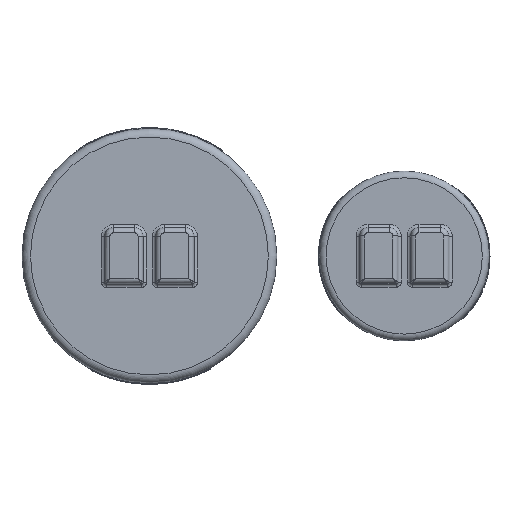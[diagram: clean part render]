
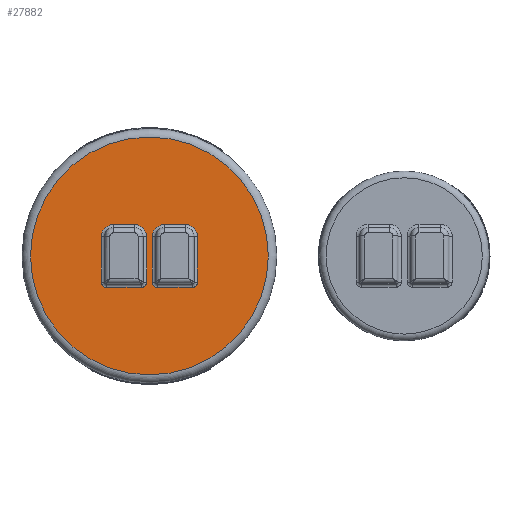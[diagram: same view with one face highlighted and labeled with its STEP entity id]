
A CAD part, top view. The second image highlights one B-rep face of the part: STEP entity #27882.
In plain terms, the highlighted planar face has unit normal (0, 0, 1).
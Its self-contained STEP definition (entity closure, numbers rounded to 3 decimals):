
#3316=FACE_BOUND('',#9538,.T.);
#3317=FACE_BOUND('',#9539,.T.);
#3658=PLANE('',#29710);
#4695=LINE('',#64399,#6189);
#4697=LINE('',#64411,#6191);
#4699=LINE('',#64423,#6193);
#4700=LINE('',#64431,#6194);
#4709=LINE('',#64458,#6203);
#4710=LINE('',#64462,#6204);
#4711=LINE('',#64466,#6205);
#4712=LINE('',#64469,#6206);
#6189=VECTOR('',#33431,10.);
#6191=VECTOR('',#33445,10.);
#6193=VECTOR('',#33459,10.);
#6194=VECTOR('',#33470,10.);
#6203=VECTOR('',#33497,10.);
#6204=VECTOR('',#33500,10.);
#6205=VECTOR('',#33503,10.);
#6206=VECTOR('',#33506,10.);
#7891=FACE_OUTER_BOUND('',#9537,.T.);
#9537=EDGE_LOOP('',(#22693));
#9538=EDGE_LOOP('',(#22694,#22695,#22696,#22697,#22698,#22699,#22700,#22701));
#9539=EDGE_LOOP('',(#22702,#22703,#22704,#22705,#22706,#22707,#22708,#22709));
#10638=CIRCLE('',#29682,7.);
#10644=CIRCLE('',#29690,7.);
#10648=CIRCLE('',#29696,3.);
#10652=CIRCLE('',#29702,3.);
#10655=CIRCLE('',#29711,70.);
#10656=CIRCLE('',#29712,7.);
#10657=CIRCLE('',#29713,3.);
#10658=CIRCLE('',#29714,3.);
#10659=CIRCLE('',#29715,7.);
#12360=VERTEX_POINT('',#64387);
#12361=VERTEX_POINT('',#64389);
#12363=VERTEX_POINT('',#64395);
#12365=VERTEX_POINT('',#64401);
#12367=VERTEX_POINT('',#64407);
#12369=VERTEX_POINT('',#64413);
#12371=VERTEX_POINT('',#64419);
#12373=VERTEX_POINT('',#64425);
#12380=VERTEX_POINT('',#64452);
#12381=VERTEX_POINT('',#64454);
#12382=VERTEX_POINT('',#64455);
#12383=VERTEX_POINT('',#64457);
#12384=VERTEX_POINT('',#64459);
#12385=VERTEX_POINT('',#64461);
#12386=VERTEX_POINT('',#64463);
#12387=VERTEX_POINT('',#64465);
#12388=VERTEX_POINT('',#64467);
#16025=EDGE_CURVE('',#12360,#12361,#10638,.T.);
#16030=EDGE_CURVE('',#12361,#12363,#4695,.T.);
#16033=EDGE_CURVE('',#12363,#12365,#10644,.T.);
#16036=EDGE_CURVE('',#12365,#12367,#4697,.T.);
#16039=EDGE_CURVE('',#12367,#12369,#10648,.T.);
#16042=EDGE_CURVE('',#12369,#12371,#4699,.T.);
#16045=EDGE_CURVE('',#12371,#12373,#10652,.T.);
#16046=EDGE_CURVE('',#12373,#12360,#4700,.T.);
#16057=EDGE_CURVE('',#12380,#12380,#10655,.T.);
#16058=EDGE_CURVE('',#12381,#12382,#10656,.T.);
#16059=EDGE_CURVE('',#12383,#12381,#4709,.T.);
#16060=EDGE_CURVE('',#12384,#12383,#10657,.T.);
#16061=EDGE_CURVE('',#12385,#12384,#4710,.T.);
#16062=EDGE_CURVE('',#12386,#12385,#10658,.T.);
#16063=EDGE_CURVE('',#12387,#12386,#4711,.T.);
#16064=EDGE_CURVE('',#12388,#12387,#10659,.T.);
#16065=EDGE_CURVE('',#12382,#12388,#4712,.T.);
#22693=ORIENTED_EDGE('',*,*,#16057,.F.);
#22694=ORIENTED_EDGE('',*,*,#16058,.F.);
#22695=ORIENTED_EDGE('',*,*,#16059,.F.);
#22696=ORIENTED_EDGE('',*,*,#16060,.F.);
#22697=ORIENTED_EDGE('',*,*,#16061,.F.);
#22698=ORIENTED_EDGE('',*,*,#16062,.F.);
#22699=ORIENTED_EDGE('',*,*,#16063,.F.);
#22700=ORIENTED_EDGE('',*,*,#16064,.F.);
#22701=ORIENTED_EDGE('',*,*,#16065,.F.);
#22702=ORIENTED_EDGE('',*,*,#16025,.F.);
#22703=ORIENTED_EDGE('',*,*,#16046,.F.);
#22704=ORIENTED_EDGE('',*,*,#16045,.F.);
#22705=ORIENTED_EDGE('',*,*,#16042,.F.);
#22706=ORIENTED_EDGE('',*,*,#16039,.F.);
#22707=ORIENTED_EDGE('',*,*,#16036,.F.);
#22708=ORIENTED_EDGE('',*,*,#16033,.F.);
#22709=ORIENTED_EDGE('',*,*,#16030,.F.);
#27882=ADVANCED_FACE('',(#7891,#3316,#3317),#3658,.T.);
#29682=AXIS2_PLACEMENT_3D('',#64390,#33420,#33421);
#29690=AXIS2_PLACEMENT_3D('',#64405,#33438,#33439);
#29696=AXIS2_PLACEMENT_3D('',#64417,#33452,#33453);
#29702=AXIS2_PLACEMENT_3D('',#64429,#33466,#33467);
#29710=AXIS2_PLACEMENT_3D('',#64451,#33491,#33492);
#29711=AXIS2_PLACEMENT_3D('',#64453,#33493,#33494);
#29712=AXIS2_PLACEMENT_3D('',#64456,#33495,#33496);
#29713=AXIS2_PLACEMENT_3D('',#64460,#33498,#33499);
#29714=AXIS2_PLACEMENT_3D('',#64464,#33501,#33502);
#29715=AXIS2_PLACEMENT_3D('',#64468,#33504,#33505);
#33420=DIRECTION('center_axis',(0.,0.,1.));
#33421=DIRECTION('ref_axis',(0.707,0.707,0.));
#33431=DIRECTION('',(-1.,0.,0.));
#33438=DIRECTION('center_axis',(0.,0.,1.));
#33439=DIRECTION('ref_axis',(-0.707,0.707,0.));
#33445=DIRECTION('',(0.,-1.,0.));
#33452=DIRECTION('center_axis',(0.,0.,1.));
#33453=DIRECTION('ref_axis',(-0.707,-0.707,0.));
#33459=DIRECTION('',(1.,0.,0.));
#33466=DIRECTION('center_axis',(0.,0.,1.));
#33467=DIRECTION('ref_axis',(0.707,-0.707,0.));
#33470=DIRECTION('',(0.,1.,0.));
#33491=DIRECTION('center_axis',(0.,0.,1.));
#33492=DIRECTION('ref_axis',(1.,0.,0.));
#33493=DIRECTION('center_axis',(0.,0.,-1.));
#33494=DIRECTION('ref_axis',(1.,0.,0.));
#33495=DIRECTION('center_axis',(0.,0.,1.));
#33496=DIRECTION('ref_axis',(0.707,0.707,0.));
#33497=DIRECTION('',(0.,1.,0.));
#33498=DIRECTION('center_axis',(0.,0.,1.));
#33499=DIRECTION('ref_axis',(0.707,-0.707,0.));
#33500=DIRECTION('',(1.,0.,0.));
#33501=DIRECTION('center_axis',(0.,0.,1.));
#33502=DIRECTION('ref_axis',(-0.707,-0.707,0.));
#33503=DIRECTION('',(0.,-1.,0.));
#33504=DIRECTION('center_axis',(0.,0.,1.));
#33505=DIRECTION('ref_axis',(-0.707,0.707,0.));
#33506=DIRECTION('',(-1.,0.,0.));
#64387=CARTESIAN_POINT('',(-1.7,11.5,40.));
#64389=CARTESIAN_POINT('',(-8.7,18.5,40.));
#64390=CARTESIAN_POINT('Origin',(-8.7,11.5,40.));
#64395=CARTESIAN_POINT('',(-21.3,18.5,40.));
#64399=CARTESIAN_POINT('',(-1.85,18.5,40.));
#64401=CARTESIAN_POINT('',(-28.3,11.5,40.));
#64405=CARTESIAN_POINT('Origin',(-21.3,11.5,40.));
#64407=CARTESIAN_POINT('',(-28.3,-15.5,40.));
#64411=CARTESIAN_POINT('',(-28.3,8.25,40.));
#64413=CARTESIAN_POINT('',(-25.3,-18.5,40.));
#64417=CARTESIAN_POINT('Origin',(-25.3,-15.5,40.));
#64419=CARTESIAN_POINT('',(-4.7,-18.5,40.));
#64423=CARTESIAN_POINT('',(-13.15,-18.5,40.));
#64425=CARTESIAN_POINT('',(-1.7,-15.5,40.));
#64429=CARTESIAN_POINT('Origin',(-4.7,-15.5,40.));
#64431=CARTESIAN_POINT('',(-1.7,-8.25,40.));
#64451=CARTESIAN_POINT('Origin',(0.,0.,40.));
#64452=CARTESIAN_POINT('',(-70.,0.,40.));
#64453=CARTESIAN_POINT('Origin',(0.,0.,40.));
#64454=CARTESIAN_POINT('',(28.3,11.5,40.));
#64455=CARTESIAN_POINT('',(21.3,18.5,40.));
#64456=CARTESIAN_POINT('Origin',(21.3,11.5,40.));
#64457=CARTESIAN_POINT('',(28.3,-15.5,40.));
#64458=CARTESIAN_POINT('',(28.3,-8.25,40.));
#64459=CARTESIAN_POINT('',(25.3,-18.5,40.));
#64460=CARTESIAN_POINT('Origin',(25.3,-15.5,40.));
#64461=CARTESIAN_POINT('',(4.7,-18.5,40.));
#64462=CARTESIAN_POINT('',(1.85,-18.5,40.));
#64463=CARTESIAN_POINT('',(1.7,-15.5,40.));
#64464=CARTESIAN_POINT('Origin',(4.7,-15.5,40.));
#64465=CARTESIAN_POINT('',(1.7,11.5,40.));
#64466=CARTESIAN_POINT('',(1.7,8.25,40.));
#64467=CARTESIAN_POINT('',(8.7,18.5,40.));
#64468=CARTESIAN_POINT('Origin',(8.7,11.5,40.));
#64469=CARTESIAN_POINT('',(13.15,18.5,40.));
